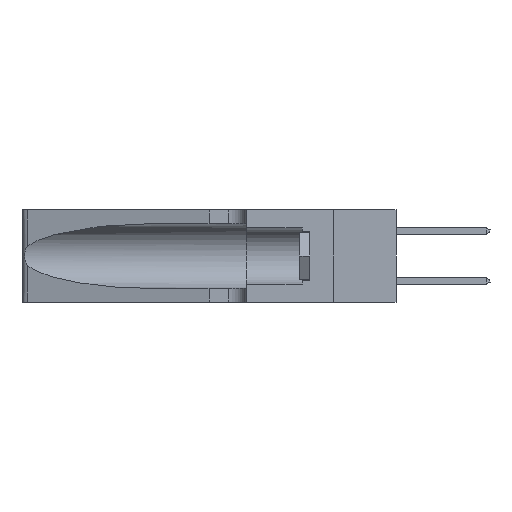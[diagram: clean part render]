
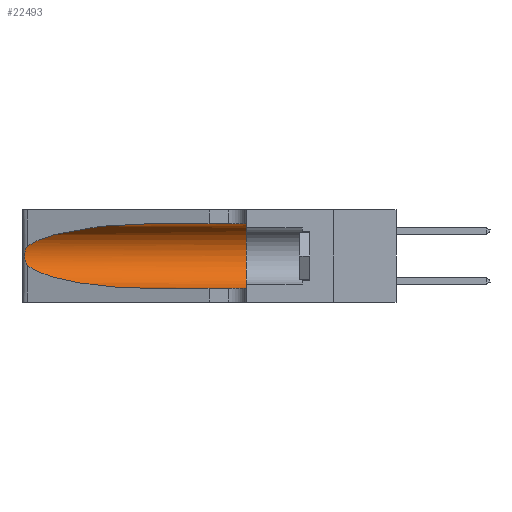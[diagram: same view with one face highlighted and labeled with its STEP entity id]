
A CAD part, left-side view. The second image highlights one B-rep face of the part: STEP entity #22493.
In plain terms, the highlighted cylindrical face has radius 3.308 mm (diameter 6.617 mm), a partial arc.
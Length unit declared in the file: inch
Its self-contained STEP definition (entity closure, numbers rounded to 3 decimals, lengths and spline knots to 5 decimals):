
#603 = CARTESIAN_POINT ( 'NONE',  ( 0.25856, 1.23593, 0.16098 ) ) ;
#936 = CARTESIAN_POINT ( 'NONE',  ( 0.25487, 1.22718, 0.22369 ) ) ;
#1357 = CARTESIAN_POINT ( 'NONE',  ( 0.2373, 1.15595, 0.08982 ) ) ;
#1695 = CARTESIAN_POINT ( 'NONE',  ( 0.1305, 0.72297, 0.05475 ) ) ;
#2587 = VERTEX_POINT ( 'NONE', #21254 ) ;
#2684 = CARTESIAN_POINT ( 'NONE',  ( 0.25487, 1.22718, 0.22369 ) ) ;
#2888 = CARTESIAN_POINT ( 'NONE',  ( 0.25639, 1.23186, 0.15144 ) ) ;
#3118 = DIRECTION ( 'NONE',  ( 0., -1., 0. ) ) ;
#3312 = ORIENTED_EDGE ( 'NONE', *, *, #24401, .F. ) ;
#4898 = VERTEX_POINT ( 'NONE', #936 ) ;
#4990 = EDGE_CURVE ( 'NONE', #8907, #24476, #6278, .T. ) ;
#5128 = LINE ( 'NONE', #27430, #22031 ) ;
#5132 = AXIS2_PLACEMENT_3D ( 'NONE', #21754, #8591, #23944 ) ;
#5144 =( BOUNDED_CURVE ( )  B_SPLINE_CURVE ( 3, ( #8153, #1357, #10400, #25746 ),
 .UNSPECIFIED., .F., .T. ) 
 B_SPLINE_CURVE_WITH_KNOTS ( ( 4, 4 ),
 ( 3.44316, 4.71239 ),
 .UNSPECIFIED. ) 
 CURVE ( )  GEOMETRIC_REPRESENTATION_ITEM ( )  RATIONAL_B_SPLINE_CURVE ( ( 1., 0.87, 0.87, 1. ) ) 
 REPRESENTATION_ITEM ( '' )  );
#5172 = CARTESIAN_POINT ( 'NONE',  ( 0.25487, 1.22718, 0.14631 ) ) ;
#5547 = VERTEX_POINT ( 'NONE', #16294 ) ;
#5787 = CARTESIAN_POINT ( 'NONE',  ( 0.1305, 1.61858, 0.05475 ) ) ;
#5866 = EDGE_CURVE ( 'NONE', #2587, #24476, #6228, .T. ) ;
#6228 = CIRCLE ( 'NONE', #5132, 0.13025 ) ;
#6278 = LINE ( 'NONE', #5787, #22462 ) ;
#7162 = ORIENTED_EDGE ( 'NONE', *, *, #27607, .T. ) ;
#7302 = CARTESIAN_POINT ( 'NONE',  ( 0.25639, 1.23184, 0.21858 ) ) ;
#7318 = CYLINDRICAL_SURFACE ( 'NONE', #13252, 0.13025 ) ;
#7572 = ORIENTED_EDGE ( 'NONE', *, *, #5866, .F. ) ;
#7623 = CARTESIAN_POINT ( 'NONE',  ( 0.1305, 1.61858, 0.185 ) ) ;
#8031 = CARTESIAN_POINT ( 'NONE',  ( 0.1305, 0.35, 0.05475 ) ) ;
#8153 = CARTESIAN_POINT ( 'NONE',  ( 0.25487, 1.22718, 0.14631 ) ) ;
#8591 = DIRECTION ( 'NONE',  ( 0., 1., 0. ) ) ;
#8707 = EDGE_LOOP ( 'NONE', ( #7162, #20987, #24120, #18325, #7572, #3312 ) ) ;
#8907 = VERTEX_POINT ( 'NONE', #1695 ) ;
#8965 = CARTESIAN_POINT ( 'NONE',  ( 0.1305, 0.72297, 0.31525 ) ) ;
#9550 = CARTESIAN_POINT ( 'NONE',  ( 0.25854, 1.2359, 0.20912 ) ) ;
#10400 = CARTESIAN_POINT ( 'NONE',  ( 0.18966, 0.96281, 0.05475 ) ) ;
#11802 = CARTESIAN_POINT ( 'NONE',  ( 0.26075, 1.23896, 0.19203 ) ) ;
#13252 = AXIS2_PLACEMENT_3D ( 'NONE', #7623, #3118, #25233 ) ;
#13407 = CARTESIAN_POINT ( 'NONE',  ( 0.2373, 1.15595, 0.28018 ) ) ;
#13994 = CARTESIAN_POINT ( 'NONE',  ( 0.26017, 1.23833, 0.17102 ) ) ;
#16182 = CARTESIAN_POINT ( 'NONE',  ( 0.25789, 1.23486, 0.15765 ) ) ;
#16294 = CARTESIAN_POINT ( 'NONE',  ( 0.25487, 1.22718, 0.14631 ) ) ;
#18157 = VERTEX_POINT ( 'NONE', #22952 ) ;
#18306 = CARTESIAN_POINT ( 'NONE',  ( 0.25487, 1.22718, 0.22369 ) ) ;
#18325 = ORIENTED_EDGE ( 'NONE', *, *, #4990, .T. ) ;
#18392 = CARTESIAN_POINT ( 'NONE',  ( 0.25555, 1.22993, 0.14849 ) ) ;
#18412 =( BOUNDED_CURVE ( )  B_SPLINE_CURVE ( 3, ( #8965, #21728, #13407, #2684 ),
 .UNSPECIFIED., .F., .F. ) 
 B_SPLINE_CURVE_WITH_KNOTS ( ( 4, 4 ),
 ( 1.5708, 2.84003 ),
 .UNSPECIFIED. ) 
 CURVE ( )  GEOMETRIC_REPRESENTATION_ITEM ( )  RATIONAL_B_SPLINE_CURVE ( ( 1., 0.87, 0.87, 1. ) ) 
 REPRESENTATION_ITEM ( '' )  );
#18702 = DIRECTION ( 'NONE',  ( 0., -1., 0. ) ) ;
#19008 = DIRECTION ( 'NONE',  ( 0., -1., 0. ) ) ;
#19047 = FACE_OUTER_BOUND ( 'NONE', #8707, .T. ) ;
#20987 = ORIENTED_EDGE ( 'NONE', *, *, #25242, .T. ) ;
#21254 = CARTESIAN_POINT ( 'NONE',  ( 0.1305, 0.35, 0.31525 ) ) ;
#21728 = CARTESIAN_POINT ( 'NONE',  ( 0.18966, 0.96281, 0.31525 ) ) ;
#21754 = CARTESIAN_POINT ( 'NONE',  ( 0.1305, 0.35, 0.185 ) ) ;
#21981 = EDGE_CURVE ( 'NONE', #5547, #8907, #5144, .T. ) ;
#22031 = VECTOR ( 'NONE', #18702, 39.37008 ) ;
#22462 = VECTOR ( 'NONE', #19008, 39.37008 ) ;
#22493 = ADVANCED_FACE ( 'NONE', ( #19047 ), #7318, .F. ) ;
#22704 = CARTESIAN_POINT ( 'NONE',  ( 0.25787, 1.23484, 0.2124 ) ) ;
#22952 = CARTESIAN_POINT ( 'NONE',  ( 0.1305, 0.72297, 0.31525 ) ) ;
#23502 = B_SPLINE_CURVE_WITH_KNOTS ( 'NONE', 3,
 ( #18306, #24829, #7302, #22704, #9550, #24918, #11802, #27112, #13994, #603, #16182, #2888, #18392, #5172 ),
 .UNSPECIFIED., .F., .F.,
 ( 4, 2, 2, 2, 2, 2, 4 ),
 ( 0., 0.00027, 0.00053, 0.00107, 0.0016, 0.00187, 0.00214 ),
 .UNSPECIFIED. ) ;
#23944 = DIRECTION ( 'NONE',  ( 0., 0., 1. ) ) ;
#24120 = ORIENTED_EDGE ( 'NONE', *, *, #21981, .T. ) ;
#24401 = EDGE_CURVE ( 'NONE', #18157, #2587, #5128, .T. ) ;
#24476 = VERTEX_POINT ( 'NONE', #8031 ) ;
#24829 = CARTESIAN_POINT ( 'NONE',  ( 0.25555, 1.22994, 0.2215 ) ) ;
#24918 = CARTESIAN_POINT ( 'NONE',  ( 0.26018, 1.23835, 0.19895 ) ) ;
#25233 = DIRECTION ( 'NONE',  ( 0., 0., -1. ) ) ;
#25242 = EDGE_CURVE ( 'NONE', #4898, #5547, #23502, .T. ) ;
#25746 = CARTESIAN_POINT ( 'NONE',  ( 0.1305, 0.72297, 0.05475 ) ) ;
#27112 = CARTESIAN_POINT ( 'NONE',  ( 0.26075, 1.23896, 0.178 ) ) ;
#27430 = CARTESIAN_POINT ( 'NONE',  ( 0.1305, 1.61858, 0.31525 ) ) ;
#27607 = EDGE_CURVE ( 'NONE', #18157, #4898, #18412, .T. ) ;
